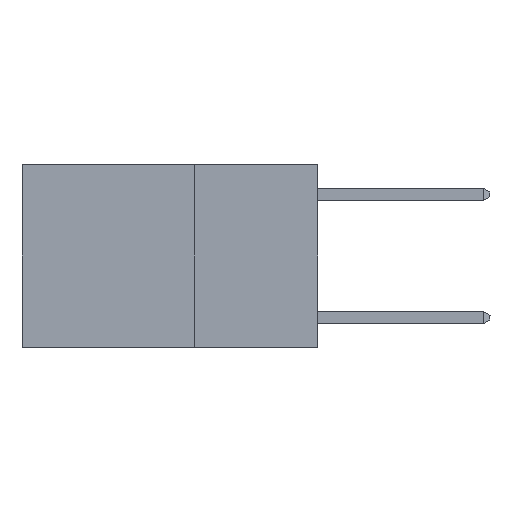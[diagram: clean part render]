
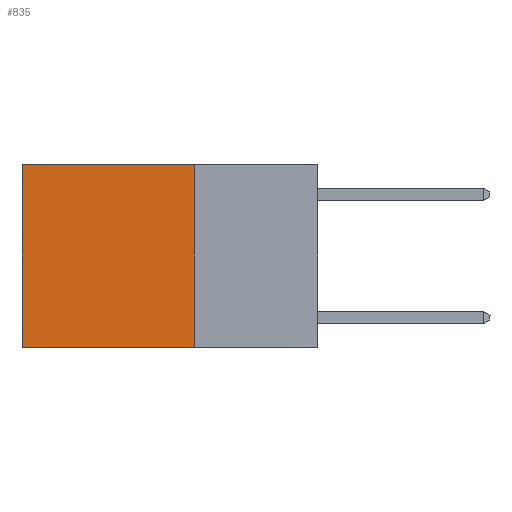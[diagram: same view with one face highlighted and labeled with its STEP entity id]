
A CAD part, left-side view. The second image highlights one B-rep face of the part: STEP entity #835.
In plain terms, the highlighted planar face has unit normal (-1, 0, 0).
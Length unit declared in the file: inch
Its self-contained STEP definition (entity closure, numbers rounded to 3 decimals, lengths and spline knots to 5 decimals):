
#517 = EDGE_CURVE ( 'NONE', #16576, #16220, #7570, .T. ) ;
#635 = CARTESIAN_POINT ( 'NONE',  ( 0.2625, 0.25, 0. ) ) ;
#835 = ADVANCED_FACE ( 'NONE', ( #1134 ), #2226, .F. ) ;
#1134 = FACE_OUTER_BOUND ( 'NONE', #9874, .T. ) ;
#1468 = EDGE_CURVE ( 'NONE', #14238, #22268, #7862, .T. ) ;
#1595 = AXIS2_PLACEMENT_3D ( 'NONE', #635, #13681, #8532 ) ;
#2226 = PLANE ( 'NONE',  #1595 ) ;
#2354 = VECTOR ( 'NONE', #7515, 39.37008 ) ;
#2471 = EDGE_CURVE ( 'NONE', #16220, #22268, #10602, .T. ) ;
#2661 = VECTOR ( 'NONE', #6451, 39.37008 ) ;
#2678 = CARTESIAN_POINT ( 'NONE',  ( 0.2625, 0.6, -0.37 ) ) ;
#5544 = CARTESIAN_POINT ( 'NONE',  ( 0.2625, 0.25, -0.37 ) ) ;
#6451 = DIRECTION ( 'NONE',  ( 0., 0., -1. ) ) ;
#7515 = DIRECTION ( 'NONE',  ( 0., 1., 0. ) ) ;
#7570 = LINE ( 'NONE', #12388, #22806 ) ;
#7862 = LINE ( 'NONE', #14122, #2661 ) ;
#8431 = CARTESIAN_POINT ( 'NONE',  ( 0.2625, 0.25, 0. ) ) ;
#8532 = DIRECTION ( 'NONE',  ( 0., 0., -1. ) ) ;
#8986 = ORIENTED_EDGE ( 'NONE', *, *, #517, .F. ) ;
#9669 = DIRECTION ( 'NONE',  ( 0., 1., 0. ) ) ;
#9727 = ORIENTED_EDGE ( 'NONE', *, *, #1468, .T. ) ;
#9874 = EDGE_LOOP ( 'NONE', ( #9727, #21390, #8986, #19708 ) ) ;
#10602 = LINE ( 'NONE', #11599, #15107 ) ;
#11599 = CARTESIAN_POINT ( 'NONE',  ( 0.2625, 0.25, -0.37 ) ) ;
#12213 = EDGE_CURVE ( 'NONE', #16576, #14238, #17185, .T. ) ;
#12388 = CARTESIAN_POINT ( 'NONE',  ( 0.2625, 0.25, 0. ) ) ;
#13681 = DIRECTION ( 'NONE',  ( 1., 0., 0. ) ) ;
#14122 = CARTESIAN_POINT ( 'NONE',  ( 0.2625, 0.6, 0. ) ) ;
#14238 = VERTEX_POINT ( 'NONE', #15070 ) ;
#15070 = CARTESIAN_POINT ( 'NONE',  ( 0.2625, 0.6, 0. ) ) ;
#15107 = VECTOR ( 'NONE', #9669, 39.37008 ) ;
#16220 = VERTEX_POINT ( 'NONE', #5544 ) ;
#16576 = VERTEX_POINT ( 'NONE', #8431 ) ;
#17185 = LINE ( 'NONE', #18985, #2354 ) ;
#18985 = CARTESIAN_POINT ( 'NONE',  ( 0.2625, 0.25, 0. ) ) ;
#19708 = ORIENTED_EDGE ( 'NONE', *, *, #12213, .T. ) ;
#21390 = ORIENTED_EDGE ( 'NONE', *, *, #2471, .F. ) ;
#22268 = VERTEX_POINT ( 'NONE', #2678 ) ;
#22806 = VECTOR ( 'NONE', #24629, 39.37008 ) ;
#24629 = DIRECTION ( 'NONE',  ( 0., 0., -1. ) ) ;
